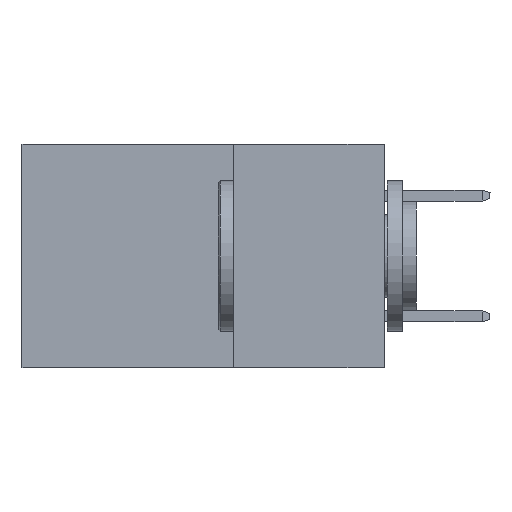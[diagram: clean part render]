
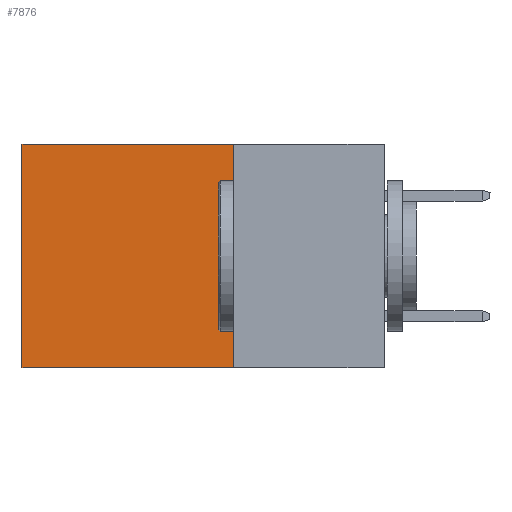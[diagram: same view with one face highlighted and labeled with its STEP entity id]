
A CAD part, left-side view. The second image highlights one B-rep face of the part: STEP entity #7876.
In plain terms, the highlighted planar face has unit normal (-1, 0, 0).
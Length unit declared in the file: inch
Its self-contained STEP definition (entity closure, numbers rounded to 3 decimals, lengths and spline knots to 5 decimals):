
#105 = DIRECTION ( 'NONE',  ( 0., 0., -1. ) ) ;
#268 = LINE ( 'NONE', #3616, #20703 ) ;
#2754 = EDGE_CURVE ( 'NONE', #15374, #10317, #17634, .T. ) ;
#3616 = CARTESIAN_POINT ( 'NONE',  ( 0.298, 0.6, 0. ) ) ;
#4227 = CARTESIAN_POINT ( 'NONE',  ( 0.298, 0.25, -0.37 ) ) ;
#5181 = LINE ( 'NONE', #19509, #8349 ) ;
#5248 = EDGE_LOOP ( 'NONE', ( #10718, #5454, #8703, #15688 ) ) ;
#5454 = ORIENTED_EDGE ( 'NONE', *, *, #20580, .F. ) ;
#5520 = LINE ( 'NONE', #4227, #13984 ) ;
#5836 = DIRECTION ( 'NONE',  ( 0., 0., -1. ) ) ;
#6094 = DIRECTION ( 'NONE',  ( 0., 1., 0. ) ) ;
#6800 = EDGE_CURVE ( 'NONE', #15374, #9870, #5181, .T. ) ;
#7876 = ADVANCED_FACE ( 'NONE', ( #12513 ), #20362, .F. ) ;
#8337 = CARTESIAN_POINT ( 'NONE',  ( 0.298, 0.6, -0.37 ) ) ;
#8349 = VECTOR ( 'NONE', #6094, 39.37008 ) ;
#8703 = ORIENTED_EDGE ( 'NONE', *, *, #2754, .F. ) ;
#8993 = VECTOR ( 'NONE', #105, 39.37008 ) ;
#9121 = DIRECTION ( 'NONE',  ( 1., 0., 0. ) ) ;
#9234 = CARTESIAN_POINT ( 'NONE',  ( 0.298, 0.6, 0. ) ) ;
#9347 = DIRECTION ( 'NONE',  ( 0., 1., 0. ) ) ;
#9870 = VERTEX_POINT ( 'NONE', #9234 ) ;
#10317 = VERTEX_POINT ( 'NONE', #13778 ) ;
#10718 = ORIENTED_EDGE ( 'NONE', *, *, #16563, .T. ) ;
#11392 = CARTESIAN_POINT ( 'NONE',  ( 0.298, 0.25, 0. ) ) ;
#12198 = AXIS2_PLACEMENT_3D ( 'NONE', #14186, #9121, #5836 ) ;
#12513 = FACE_OUTER_BOUND ( 'NONE', #5248, .T. ) ;
#13778 = CARTESIAN_POINT ( 'NONE',  ( 0.298, 0.25, -0.37 ) ) ;
#13984 = VECTOR ( 'NONE', #9347, 39.37008 ) ;
#14186 = CARTESIAN_POINT ( 'NONE',  ( 0.298, 0.25, 0. ) ) ;
#15374 = VERTEX_POINT ( 'NONE', #15997 ) ;
#15688 = ORIENTED_EDGE ( 'NONE', *, *, #6800, .T. ) ;
#15997 = CARTESIAN_POINT ( 'NONE',  ( 0.298, 0.25, 0. ) ) ;
#16563 = EDGE_CURVE ( 'NONE', #9870, #21493, #268, .T. ) ;
#17031 = DIRECTION ( 'NONE',  ( 0., 0., -1. ) ) ;
#17634 = LINE ( 'NONE', #11392, #8993 ) ;
#19509 = CARTESIAN_POINT ( 'NONE',  ( 0.298, 0.25, 0. ) ) ;
#20362 = PLANE ( 'NONE',  #12198 ) ;
#20580 = EDGE_CURVE ( 'NONE', #10317, #21493, #5520, .T. ) ;
#20703 = VECTOR ( 'NONE', #17031, 39.37008 ) ;
#21493 = VERTEX_POINT ( 'NONE', #8337 ) ;
